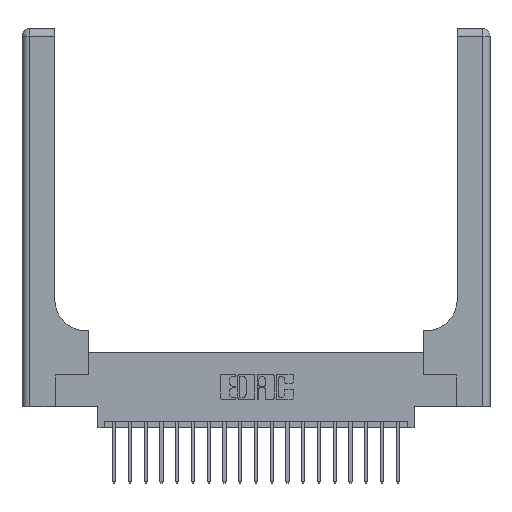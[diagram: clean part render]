
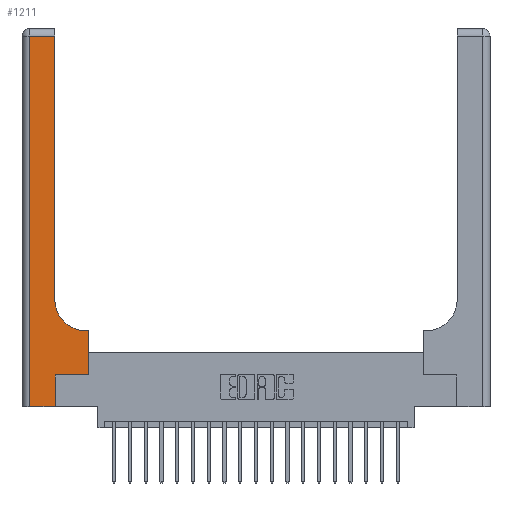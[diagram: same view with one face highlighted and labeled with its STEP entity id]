
A CAD part, top view. The second image highlights one B-rep face of the part: STEP entity #1211.
In plain terms, the highlighted planar face has unit normal (0, 0, 1).
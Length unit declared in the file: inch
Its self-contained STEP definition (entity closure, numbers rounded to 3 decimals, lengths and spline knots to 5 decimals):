
#161 = VERTEX_POINT ( 'NONE', #4472 ) ;
#481 = VERTEX_POINT ( 'NONE', #18010 ) ;
#510 = VERTEX_POINT ( 'NONE', #6853 ) ;
#814 = LINE ( 'NONE', #4854, #17454 ) ;
#1121 = VECTOR ( 'NONE', #5032, 39.37008 ) ;
#1211 = ADVANCED_FACE ( 'NONE', ( #18851 ), #10311, .F. ) ;
#1282 = LINE ( 'NONE', #15885, #9393 ) ;
#2289 = DIRECTION ( 'NONE',  ( 0., 0., -1. ) ) ;
#2343 = VECTOR ( 'NONE', #20148, 39.37008 ) ;
#3318 = VECTOR ( 'NONE', #14640, 39.37008 ) ;
#3532 = ORIENTED_EDGE ( 'NONE', *, *, #16772, .T. ) ;
#3649 = EDGE_CURVE ( 'NONE', #12646, #161, #10761, .T. ) ;
#4145 = CARTESIAN_POINT ( 'NONE',  ( 0.51, 0.6, 0.37 ) ) ;
#4167 = VECTOR ( 'NONE', #6881, 39.37008 ) ;
#4472 = CARTESIAN_POINT ( 'NONE',  ( 0.265, 0., 0.37 ) ) ;
#4814 = CARTESIAN_POINT ( 'NONE',  ( 0.26, 0.6, 0.37 ) ) ;
#4854 = CARTESIAN_POINT ( 'NONE',  ( 0.26, 3., 0.37 ) ) ;
#5032 = DIRECTION ( 'NONE',  ( 1., 0., 0. ) ) ;
#5261 = CARTESIAN_POINT ( 'NONE',  ( 0.265, 0.25, 0.37 ) ) ;
#5381 = ORIENTED_EDGE ( 'NONE', *, *, #20251, .T. ) ;
#5405 = CARTESIAN_POINT ( 'NONE',  ( 0., 3., 0.37 ) ) ;
#5949 = ORIENTED_EDGE ( 'NONE', *, *, #15619, .T. ) ;
#6293 = VECTOR ( 'NONE', #9218, 39.37008 ) ;
#6406 = ORIENTED_EDGE ( 'NONE', *, *, #12822, .T. ) ;
#6476 = DIRECTION ( 'NONE',  ( 0., 1., 0. ) ) ;
#6581 = LINE ( 'NONE', #8188, #3318 ) ;
#6853 = CARTESIAN_POINT ( 'NONE',  ( 0.528, 0.25, 0.37 ) ) ;
#6881 = DIRECTION ( 'NONE',  ( 1., 0., 0. ) ) ;
#7113 = DIRECTION ( 'NONE',  ( -1., 0., 0. ) ) ;
#7130 = VECTOR ( 'NONE', #11271, 39.37008 ) ;
#7431 = CARTESIAN_POINT ( 'NONE',  ( 0.265, 0.25, 0.37 ) ) ;
#7903 = DIRECTION ( 'NONE',  ( 0., -1., 0. ) ) ;
#8188 = CARTESIAN_POINT ( 'NONE',  ( 0., 2.94, 0.37 ) ) ;
#8538 = VERTEX_POINT ( 'NONE', #17600 ) ;
#8964 = CARTESIAN_POINT ( 'NONE',  ( 0.265, 0., 0.37 ) ) ;
#8996 = LINE ( 'NONE', #5261, #4167 ) ;
#9218 = DIRECTION ( 'NONE',  ( 0., 1., 0. ) ) ;
#9393 = VECTOR ( 'NONE', #7903, 39.37008 ) ;
#9759 = EDGE_CURVE ( 'NONE', #12587, #17337, #16162, .T. ) ;
#10311 = PLANE ( 'NONE',  #17918 ) ;
#10318 = VERTEX_POINT ( 'NONE', #14592 ) ;
#10613 = LINE ( 'NONE', #20403, #6293 ) ;
#10761 = LINE ( 'NONE', #11477, #1121 ) ;
#10843 = EDGE_CURVE ( 'NONE', #481, #12646, #1282, .T. ) ;
#10947 = EDGE_CURVE ( 'NONE', #17337, #8538, #15875, .T. ) ;
#11271 = DIRECTION ( 'NONE',  ( -1., 0., 0. ) ) ;
#11471 = LINE ( 'NONE', #8964, #2343 ) ;
#11477 = CARTESIAN_POINT ( 'NONE',  ( 0., 0., 0.37 ) ) ;
#11727 = ORIENTED_EDGE ( 'NONE', *, *, #10843, .T. ) ;
#11963 = CARTESIAN_POINT ( 'NONE',  ( 0.51, 0.85, 0.37 ) ) ;
#12587 = VERTEX_POINT ( 'NONE', #19191 ) ;
#12646 = VERTEX_POINT ( 'NONE', #17707 ) ;
#12822 = EDGE_CURVE ( 'NONE', #13607, #510, #8996, .T. ) ;
#12997 = EDGE_LOOP ( 'NONE', ( #5381, #5949, #11727, #19242, #18942, #6406, #3532, #14903, #13092 ) ) ;
#13092 = ORIENTED_EDGE ( 'NONE', *, *, #10947, .T. ) ;
#13574 = DIRECTION ( 'NONE',  ( 1., 0., 0. ) ) ;
#13607 = VERTEX_POINT ( 'NONE', #7431 ) ;
#14143 = EDGE_CURVE ( 'NONE', #161, #13607, #11471, .T. ) ;
#14592 = CARTESIAN_POINT ( 'NONE',  ( 0.26, 2.94, 0.37 ) ) ;
#14640 = DIRECTION ( 'NONE',  ( -1., 0., 0. ) ) ;
#14903 = ORIENTED_EDGE ( 'NONE', *, *, #9759, .T. ) ;
#15619 = EDGE_CURVE ( 'NONE', #10318, #481, #6581, .T. ) ;
#15875 = CIRCLE ( 'NONE', #20343, 0.25 ) ;
#15885 = CARTESIAN_POINT ( 'NONE',  ( 0.06, 3., 0.37 ) ) ;
#16162 = LINE ( 'NONE', #4814, #7130 ) ;
#16718 = DIRECTION ( 'NONE',  ( 0., 0., -1. ) ) ;
#16772 = EDGE_CURVE ( 'NONE', #510, #12587, #10613, .T. ) ;
#17337 = VERTEX_POINT ( 'NONE', #4145 ) ;
#17454 = VECTOR ( 'NONE', #6476, 39.37008 ) ;
#17600 = CARTESIAN_POINT ( 'NONE',  ( 0.26, 0.85, 0.37 ) ) ;
#17707 = CARTESIAN_POINT ( 'NONE',  ( 0.06, 0., 0.37 ) ) ;
#17918 = AXIS2_PLACEMENT_3D ( 'NONE', #5405, #16718, #7113 ) ;
#18010 = CARTESIAN_POINT ( 'NONE',  ( 0.06, 2.94, 0.37 ) ) ;
#18851 = FACE_OUTER_BOUND ( 'NONE', #12997, .T. ) ;
#18942 = ORIENTED_EDGE ( 'NONE', *, *, #14143, .T. ) ;
#19191 = CARTESIAN_POINT ( 'NONE',  ( 0.528, 0.6, 0.37 ) ) ;
#19242 = ORIENTED_EDGE ( 'NONE', *, *, #3649, .T. ) ;
#20148 = DIRECTION ( 'NONE',  ( 0., 1., 0. ) ) ;
#20251 = EDGE_CURVE ( 'NONE', #8538, #10318, #814, .T. ) ;
#20343 = AXIS2_PLACEMENT_3D ( 'NONE', #11963, #2289, #13574 ) ;
#20403 = CARTESIAN_POINT ( 'NONE',  ( 0.528, 0.25, 0.37 ) ) ;
